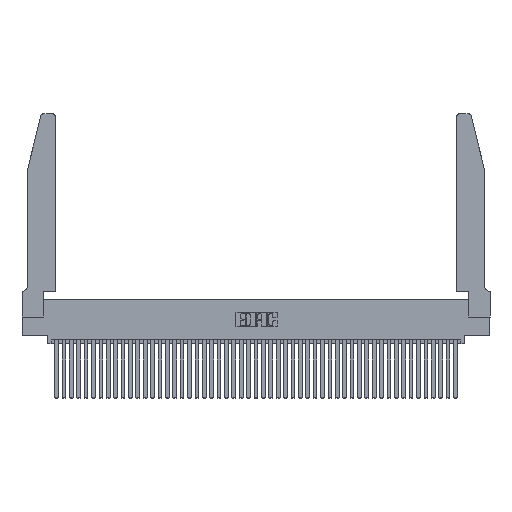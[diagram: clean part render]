
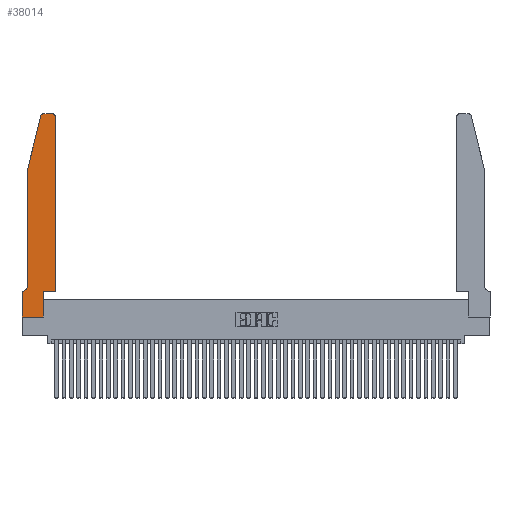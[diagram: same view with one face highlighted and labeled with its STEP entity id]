
A CAD part, top view. The second image highlights one B-rep face of the part: STEP entity #38014.
In plain terms, the highlighted planar face has unit normal (0, 0, 1).
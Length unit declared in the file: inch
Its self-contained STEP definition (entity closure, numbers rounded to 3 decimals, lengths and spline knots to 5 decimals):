
#392 = ORIENTED_EDGE ( 'NONE', *, *, #44478, .T. ) ;
#603 = LINE ( 'NONE', #19765, #21776 ) ;
#699 = DIRECTION ( 'NONE',  ( -1., 0., 0. ) ) ;
#718 = DIRECTION ( 'NONE',  ( -0.239, -0.971, 0. ) ) ;
#998 = CARTESIAN_POINT ( 'NONE',  ( 0., 0.35, 0.37 ) ) ;
#1461 = DIRECTION ( 'NONE',  ( 0., 0., 1. ) ) ;
#2859 = CIRCLE ( 'NONE', #31024, 0.03 ) ;
#3437 = CARTESIAN_POINT ( 'NONE',  ( 0.4505, 0.35, 0.37 ) ) ;
#4435 = EDGE_CURVE ( 'NONE', #19957, #18144, #2859, .T. ) ;
#4922 = VECTOR ( 'NONE', #8226, 39.37008 ) ;
#5833 = CARTESIAN_POINT ( 'NONE',  ( 0., 0., 0.37 ) ) ;
#6205 = VERTEX_POINT ( 'NONE', #41759 ) ;
#6221 = ORIENTED_EDGE ( 'NONE', *, *, #31753, .T. ) ;
#6710 = VECTOR ( 'NONE', #7063, 39.37008 ) ;
#7063 = DIRECTION ( 'NONE',  ( 0., 1., 0. ) ) ;
#7397 = EDGE_CURVE ( 'NONE', #42902, #6205, #26114, .T. ) ;
#7803 = ORIENTED_EDGE ( 'NONE', *, *, #10505, .T. ) ;
#8226 = DIRECTION ( 'NONE',  ( 1., 0., 0. ) ) ;
#8541 = EDGE_CURVE ( 'NONE', #35622, #41324, #19263, .T. ) ;
#8685 = FACE_OUTER_BOUND ( 'NONE', #10384, .T. ) ;
#9049 = AXIS2_PLACEMENT_3D ( 'NONE', #26127, #15181, #11917 ) ;
#9786 = DIRECTION ( 'NONE',  ( 1., 0., 0. ) ) ;
#9853 = CARTESIAN_POINT ( 'NONE',  ( 0.2865, 0.35, 0.37 ) ) ;
#10171 = DIRECTION ( 'NONE',  ( 0., 1., 0. ) ) ;
#10384 = EDGE_LOOP ( 'NONE', ( #18850, #32838, #6221, #45525, #36684, #392, #7803, #33968, #29724, #36775, #21829, #38937 ) ) ;
#10505 = EDGE_CURVE ( 'NONE', #26030, #35622, #38086, .T. ) ;
#10999 = VERTEX_POINT ( 'NONE', #3437 ) ;
#11117 = CARTESIAN_POINT ( 'NONE',  ( 0.2865, 0.35, 0.37 ) ) ;
#11266 = EDGE_CURVE ( 'NONE', #41324, #27216, #27378, .T. ) ;
#11917 = DIRECTION ( 'NONE',  ( -1., 0., 0. ) ) ;
#11976 = DIRECTION ( 'NONE',  ( -1., 0., 0. ) ) ;
#13379 = CARTESIAN_POINT ( 'NONE',  ( 0.284, 2.72, 0.37 ) ) ;
#14115 = PLANE ( 'NONE',  #36382 ) ;
#14523 = CIRCLE ( 'NONE', #41316, 0.03 ) ;
#15074 = VECTOR ( 'NONE', #10171, 39.37008 ) ;
#15181 = DIRECTION ( 'NONE',  ( 0., 0., -1. ) ) ;
#15225 = CARTESIAN_POINT ( 'NONE',  ( 0.4505, 0.35, 0.37 ) ) ;
#17019 = DIRECTION ( 'NONE',  ( 0., -1., 0. ) ) ;
#17692 = DIRECTION ( 'NONE',  ( 1., 0., 0. ) ) ;
#17759 = VERTEX_POINT ( 'NONE', #43519 ) ;
#18144 = VERTEX_POINT ( 'NONE', #37888 ) ;
#18850 = ORIENTED_EDGE ( 'NONE', *, *, #29559, .T. ) ;
#19263 = LINE ( 'NONE', #5833, #42678 ) ;
#19765 = CARTESIAN_POINT ( 'NONE',  ( 0.0755, 0.35, 0.37 ) ) ;
#19957 = VERTEX_POINT ( 'NONE', #20235 ) ;
#20235 = CARTESIAN_POINT ( 'NONE',  ( 0.4505, 2.72, 0.37 ) ) ;
#21776 = VECTOR ( 'NONE', #11976, 39.37008 ) ;
#21829 = ORIENTED_EDGE ( 'NONE', *, *, #35439, .T. ) ;
#22973 = DIRECTION ( 'NONE',  ( 0., -1., 0. ) ) ;
#23536 = LINE ( 'NONE', #39983, #25738 ) ;
#23880 = VECTOR ( 'NONE', #17019, 39.37008 ) ;
#23982 = DIRECTION ( 'NONE',  ( 0., 0., 1. ) ) ;
#24877 = CARTESIAN_POINT ( 'NONE',  ( 0., 0.35, 0.37 ) ) ;
#25255 = CARTESIAN_POINT ( 'NONE',  ( 0.0055, 0.35, 0.37 ) ) ;
#25738 = VECTOR ( 'NONE', #718, 39.37008 ) ;
#25771 = CARTESIAN_POINT ( 'NONE',  ( 0.2605, 2.75, 0.37 ) ) ;
#25777 = VECTOR ( 'NONE', #22973, 39.37008 ) ;
#26030 = VERTEX_POINT ( 'NONE', #998 ) ;
#26114 = LINE ( 'NONE', #28241, #23880 ) ;
#26127 = CARTESIAN_POINT ( 'NONE',  ( 0.0055, 0.42, 0.37 ) ) ;
#27216 = VERTEX_POINT ( 'NONE', #9853 ) ;
#27378 = LINE ( 'NONE', #11117, #15074 ) ;
#28241 = CARTESIAN_POINT ( 'NONE',  ( 0.0755, 2., 0.37 ) ) ;
#29037 = LINE ( 'NONE', #46047, #6710 ) ;
#29559 = EDGE_CURVE ( 'NONE', #18144, #17759, #37096, .T. ) ;
#29724 = ORIENTED_EDGE ( 'NONE', *, *, #11266, .T. ) ;
#30530 = DIRECTION ( 'NONE',  ( 1., 0., 0. ) ) ;
#31024 = AXIS2_PLACEMENT_3D ( 'NONE', #41013, #1461, #33413 ) ;
#31481 = DIRECTION ( 'NONE',  ( 0., 0., 1. ) ) ;
#31753 = EDGE_CURVE ( 'NONE', #45030, #42902, #23536, .T. ) ;
#32304 = CARTESIAN_POINT ( 'NONE',  ( 0.2865, 0., 0.37 ) ) ;
#32838 = ORIENTED_EDGE ( 'NONE', *, *, #44492, .T. ) ;
#33413 = DIRECTION ( 'NONE',  ( 1., 0., 0. ) ) ;
#33736 = CARTESIAN_POINT ( 'NONE',  ( 0., 0., 0.37 ) ) ;
#33968 = ORIENTED_EDGE ( 'NONE', *, *, #8541, .T. ) ;
#35149 = CARTESIAN_POINT ( 'NONE',  ( 0.0755, 2., 0.37 ) ) ;
#35439 = EDGE_CURVE ( 'NONE', #10999, #19957, #29037, .T. ) ;
#35622 = VERTEX_POINT ( 'NONE', #36889 ) ;
#36382 = AXIS2_PLACEMENT_3D ( 'NONE', #24877, #31481, #17692 ) ;
#36684 = ORIENTED_EDGE ( 'NONE', *, *, #45001, .T. ) ;
#36775 = ORIENTED_EDGE ( 'NONE', *, *, #39401, .T. ) ;
#36889 = CARTESIAN_POINT ( 'NONE',  ( 0., 0., 0.37 ) ) ;
#37096 = LINE ( 'NONE', #25771, #45426 ) ;
#37888 = CARTESIAN_POINT ( 'NONE',  ( 0.4205, 2.75, 0.37 ) ) ;
#38014 = ADVANCED_FACE ( 'NONE', ( #8685 ), #14115, .T. ) ;
#38086 = LINE ( 'NONE', #33736, #25777 ) ;
#38930 = VERTEX_POINT ( 'NONE', #25255 ) ;
#38937 = ORIENTED_EDGE ( 'NONE', *, *, #4435, .T. ) ;
#39401 = EDGE_CURVE ( 'NONE', #27216, #10999, #41154, .T. ) ;
#39983 = CARTESIAN_POINT ( 'NONE',  ( 0.0755, 2., 0.37 ) ) ;
#41013 = CARTESIAN_POINT ( 'NONE',  ( 0.4205, 2.72, 0.37 ) ) ;
#41154 = LINE ( 'NONE', #15225, #4922 ) ;
#41316 = AXIS2_PLACEMENT_3D ( 'NONE', #13379, #23982, #9786 ) ;
#41324 = VERTEX_POINT ( 'NONE', #32304 ) ;
#41759 = CARTESIAN_POINT ( 'NONE',  ( 0.0755, 0.42, 0.37 ) ) ;
#42678 = VECTOR ( 'NONE', #30530, 39.37008 ) ;
#42902 = VERTEX_POINT ( 'NONE', #35149 ) ;
#43519 = CARTESIAN_POINT ( 'NONE',  ( 0.284, 2.75, 0.37 ) ) ;
#43709 = CARTESIAN_POINT ( 'NONE',  ( 0.25487, 2.72718, 0.37 ) ) ;
#44478 = EDGE_CURVE ( 'NONE', #38930, #26030, #603, .T. ) ;
#44492 = EDGE_CURVE ( 'NONE', #17759, #45030, #14523, .T. ) ;
#45001 = EDGE_CURVE ( 'NONE', #6205, #38930, #45173, .T. ) ;
#45030 = VERTEX_POINT ( 'NONE', #43709 ) ;
#45173 = CIRCLE ( 'NONE', #9049, 0.07 ) ;
#45426 = VECTOR ( 'NONE', #699, 39.37008 ) ;
#45525 = ORIENTED_EDGE ( 'NONE', *, *, #7397, .T. ) ;
#46047 = CARTESIAN_POINT ( 'NONE',  ( 0.4505, 0.35, 0.37 ) ) ;
